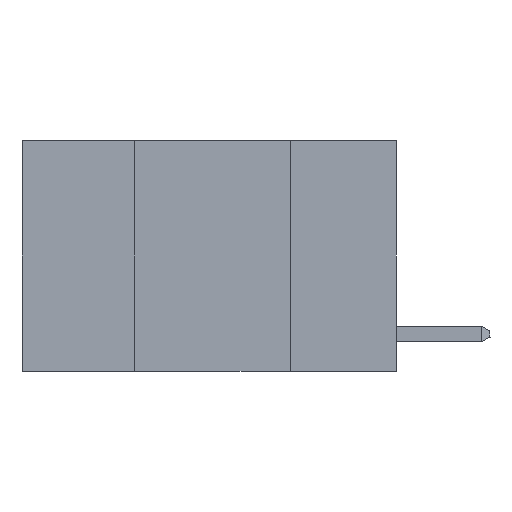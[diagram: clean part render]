
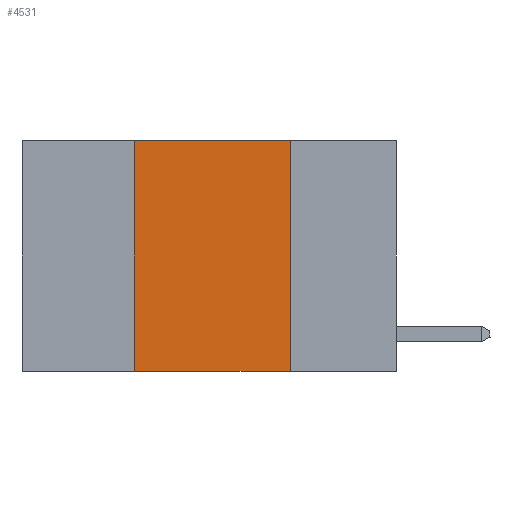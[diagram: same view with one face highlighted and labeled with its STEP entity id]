
A CAD part, left-side view. The second image highlights one B-rep face of the part: STEP entity #4531.
In plain terms, the highlighted planar face has unit normal (-1, 0, 0).
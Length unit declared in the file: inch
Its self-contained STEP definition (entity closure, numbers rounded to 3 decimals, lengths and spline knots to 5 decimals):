
#276 = CARTESIAN_POINT ( 'NONE',  ( 0., 0.6, 0. ) ) ;
#289 = ORIENTED_EDGE ( 'NONE', *, *, #9923, .F. ) ;
#675 = PLANE ( 'NONE',  #9223 ) ;
#2122 = DIRECTION ( 'NONE',  ( 0., 0., -1. ) ) ;
#2386 = LINE ( 'NONE', #9424, #3725 ) ;
#2437 = LINE ( 'NONE', #276, #5525 ) ;
#2444 = LINE ( 'NONE', #5378, #5131 ) ;
#2460 = ORIENTED_EDGE ( 'NONE', *, *, #8490, .F. ) ;
#2559 = VERTEX_POINT ( 'NONE', #7250 ) ;
#2885 = ORIENTED_EDGE ( 'NONE', *, *, #3279, .T. ) ;
#3028 = CARTESIAN_POINT ( 'NONE',  ( 0., 0.6, 0. ) ) ;
#3279 = EDGE_CURVE ( 'NONE', #4579, #8776, #2444, .T. ) ;
#3634 = CARTESIAN_POINT ( 'NONE',  ( 0., 0.17, -0.37 ) ) ;
#3725 = VECTOR ( 'NONE', #5603, 39.37008 ) ;
#4012 = DIRECTION ( 'NONE',  ( 0., -1., 0. ) ) ;
#4531 = ADVANCED_FACE ( 'NONE', ( #6712 ), #675, .F. ) ;
#4579 = VERTEX_POINT ( 'NONE', #5147 ) ;
#4864 = CARTESIAN_POINT ( 'NONE',  ( 0., 0.17, 0. ) ) ;
#5131 = VECTOR ( 'NONE', #4012, 39.37008 ) ;
#5147 = CARTESIAN_POINT ( 'NONE',  ( 0., 0.42, -0.37 ) ) ;
#5378 = CARTESIAN_POINT ( 'NONE',  ( 0., 0.6, -0.37 ) ) ;
#5453 = VERTEX_POINT ( 'NONE', #6847 ) ;
#5525 = VECTOR ( 'NONE', #6475, 39.37008 ) ;
#5603 = DIRECTION ( 'NONE',  ( 0., 0., 1. ) ) ;
#5616 = LINE ( 'NONE', #4864, #6172 ) ;
#6172 = VECTOR ( 'NONE', #8012, 39.37008 ) ;
#6475 = DIRECTION ( 'NONE',  ( 0., -1., 0. ) ) ;
#6712 = FACE_OUTER_BOUND ( 'NONE', #10038, .T. ) ;
#6847 = CARTESIAN_POINT ( 'NONE',  ( 0., 0.42, 0. ) ) ;
#7250 = CARTESIAN_POINT ( 'NONE',  ( 0., 0.17, 0. ) ) ;
#8012 = DIRECTION ( 'NONE',  ( 0., 0., -1. ) ) ;
#8490 = EDGE_CURVE ( 'NONE', #4579, #5453, #2386, .T. ) ;
#8776 = VERTEX_POINT ( 'NONE', #3634 ) ;
#9053 = ORIENTED_EDGE ( 'NONE', *, *, #9482, .F. ) ;
#9223 = AXIS2_PLACEMENT_3D ( 'NONE', #3028, #10033, #2122 ) ;
#9424 = CARTESIAN_POINT ( 'NONE',  ( 0., 0.42, 0. ) ) ;
#9482 = EDGE_CURVE ( 'NONE', #2559, #8776, #5616, .T. ) ;
#9923 = EDGE_CURVE ( 'NONE', #5453, #2559, #2437, .T. ) ;
#10033 = DIRECTION ( 'NONE',  ( 1., 0., 0. ) ) ;
#10038 = EDGE_LOOP ( 'NONE', ( #9053, #289, #2460, #2885 ) ) ;
